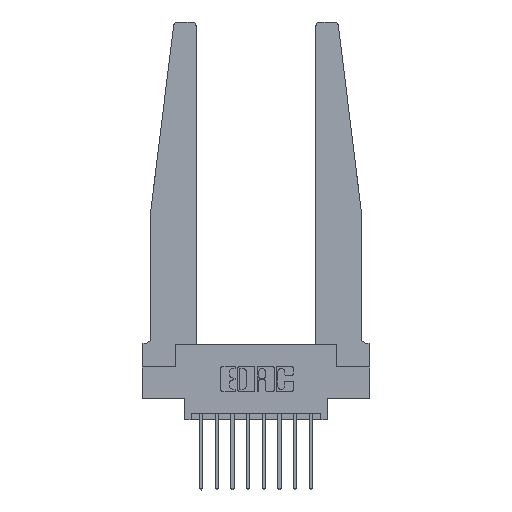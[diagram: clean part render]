
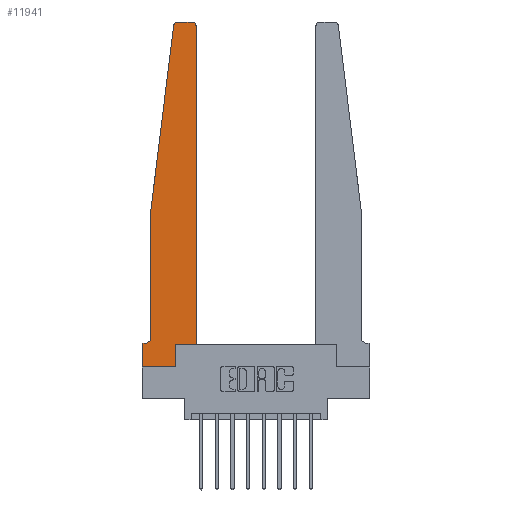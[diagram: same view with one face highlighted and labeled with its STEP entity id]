
A CAD part, top view. The second image highlights one B-rep face of the part: STEP entity #11941.
In plain terms, the highlighted planar face has unit normal (0, 0, 1).
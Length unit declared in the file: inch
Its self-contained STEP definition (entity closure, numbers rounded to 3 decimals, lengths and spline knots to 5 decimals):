
#55 = ORIENTED_EDGE ( 'NONE', *, *, #4437, .T. ) ;
#72 = VECTOR ( 'NONE', #4431, 39.37008 ) ;
#84 = VECTOR ( 'NONE', #1507, 39.37008 ) ;
#110 = CARTESIAN_POINT ( 'NONE',  ( 0.27653, 2.75, 0.37 ) ) ;
#805 = CARTESIAN_POINT ( 'NONE',  ( 0.065, 1.25, 0.37 ) ) ;
#970 = CARTESIAN_POINT ( 'NONE',  ( 0.065, 1.25, 0.37 ) ) ;
#1262 = EDGE_LOOP ( 'NONE', ( #13787, #9319, #13698, #7405, #13806, #8957, #1422, #9100, #9950, #10166, #55, #6758 ) ) ;
#1422 = ORIENTED_EDGE ( 'NONE', *, *, #10849, .T. ) ;
#1507 = DIRECTION ( 'NONE',  ( 0., 1., 0. ) ) ;
#1625 = VERTEX_POINT ( 'NONE', #13181 ) ;
#1698 = EDGE_CURVE ( 'NONE', #13795, #2586, #1751, .T. ) ;
#1751 = CIRCLE ( 'NONE', #6270, 0.05 ) ;
#2132 = AXIS2_PLACEMENT_3D ( 'NONE', #11994, #5197, #13147 ) ;
#2185 = DIRECTION ( 'NONE',  ( -1., 0., 0. ) ) ;
#2275 = LINE ( 'NONE', #2280, #10970 ) ;
#2280 = CARTESIAN_POINT ( 'NONE',  ( 0., 0., 0.37 ) ) ;
#2449 = CARTESIAN_POINT ( 'NONE',  ( 0.2605, 0.18, 0.37 ) ) ;
#2534 = VECTOR ( 'NONE', #2185, 39.37008 ) ;
#2586 = VERTEX_POINT ( 'NONE', #4735 ) ;
#2607 = DIRECTION ( 'NONE',  ( 0., 0., 1. ) ) ;
#2850 = VECTOR ( 'NONE', #12001, 39.37008 ) ;
#2880 = LINE ( 'NONE', #13566, #2534 ) ;
#3452 = CARTESIAN_POINT ( 'NONE',  ( 0., 0., 0.37 ) ) ;
#3646 = CIRCLE ( 'NONE', #10061, 0.03 ) ;
#3880 = CARTESIAN_POINT ( 'NONE',  ( 0., 0., 0.37 ) ) ;
#4180 = EDGE_CURVE ( 'NONE', #2586, #12520, #9156, .T. ) ;
#4248 = DIRECTION ( 'NONE',  ( -0.122, -0.992, 0. ) ) ;
#4431 = DIRECTION ( 'NONE',  ( -1., 0., 0. ) ) ;
#4437 = EDGE_CURVE ( 'NONE', #9619, #8622, #12184, .T. ) ;
#4735 = CARTESIAN_POINT ( 'NONE',  ( 0.015, 0.1875, 0.37 ) ) ;
#4822 = LINE ( 'NONE', #13734, #10512 ) ;
#5020 = DIRECTION ( 'NONE',  ( 0., -1., 0. ) ) ;
#5117 = LINE ( 'NONE', #3880, #11156 ) ;
#5148 = LINE ( 'NONE', #805, #10827 ) ;
#5197 = DIRECTION ( 'NONE',  ( 0., 0., 1. ) ) ;
#5408 = VERTEX_POINT ( 'NONE', #970 ) ;
#5577 = VERTEX_POINT ( 'NONE', #110 ) ;
#5584 = EDGE_CURVE ( 'NONE', #5577, #13607, #3646, .T. ) ;
#5821 = DIRECTION ( 'NONE',  ( 1., 0., 0. ) ) ;
#5870 = LINE ( 'NONE', #10859, #2850 ) ;
#5886 = DIRECTION ( 'NONE',  ( 0., 0., 1. ) ) ;
#6270 = AXIS2_PLACEMENT_3D ( 'NONE', #13327, #6499, #14466 ) ;
#6499 = DIRECTION ( 'NONE',  ( 0., 0., -1. ) ) ;
#6758 = ORIENTED_EDGE ( 'NONE', *, *, #14075, .T. ) ;
#6815 = CARTESIAN_POINT ( 'NONE',  ( 0.2605, 0.18, 0.37 ) ) ;
#6899 = VECTOR ( 'NONE', #8167, 39.37008 ) ;
#7108 = CARTESIAN_POINT ( 'NONE',  ( 0., 0.1875, 0.37 ) ) ;
#7230 = VERTEX_POINT ( 'NONE', #6815 ) ;
#7304 = CIRCLE ( 'NONE', #2132, 0.03 ) ;
#7405 = ORIENTED_EDGE ( 'NONE', *, *, #8548, .T. ) ;
#7636 = EDGE_CURVE ( 'NONE', #7230, #9619, #4822, .T. ) ;
#8167 = DIRECTION ( 'NONE',  ( 0., 1., 0. ) ) ;
#8548 = EDGE_CURVE ( 'NONE', #5408, #13795, #5870, .T. ) ;
#8622 = VERTEX_POINT ( 'NONE', #9868 ) ;
#8688 = AXIS2_PLACEMENT_3D ( 'NONE', #7108, #2607, #10537 ) ;
#8957 = ORIENTED_EDGE ( 'NONE', *, *, #4180, .T. ) ;
#9100 = ORIENTED_EDGE ( 'NONE', *, *, #11100, .T. ) ;
#9156 = LINE ( 'NONE', #12371, #72 ) ;
#9319 = ORIENTED_EDGE ( 'NONE', *, *, #5584, .T. ) ;
#9366 = CARTESIAN_POINT ( 'NONE',  ( 0., 0.1875, 0.37 ) ) ;
#9454 = CARTESIAN_POINT ( 'NONE',  ( 0.425, 0.18, 0.37 ) ) ;
#9619 = VERTEX_POINT ( 'NONE', #14051 ) ;
#9863 = EDGE_CURVE ( 'NONE', #13607, #5408, #5148, .T. ) ;
#9868 = CARTESIAN_POINT ( 'NONE',  ( 0.425, 2.72, 0.37 ) ) ;
#9935 = LINE ( 'NONE', #2449, #6899 ) ;
#9950 = ORIENTED_EDGE ( 'NONE', *, *, #10144, .T. ) ;
#10061 = AXIS2_PLACEMENT_3D ( 'NONE', #12684, #5886, #13843 ) ;
#10066 = FACE_OUTER_BOUND ( 'NONE', #1262, .T. ) ;
#10144 = EDGE_CURVE ( 'NONE', #14463, #7230, #9935, .T. ) ;
#10166 = ORIENTED_EDGE ( 'NONE', *, *, #7636, .T. ) ;
#10221 = DIRECTION ( 'NONE',  ( 1., 0., 0. ) ) ;
#10512 = VECTOR ( 'NONE', #5821, 39.37008 ) ;
#10537 = DIRECTION ( 'NONE',  ( 1., 0., 0. ) ) ;
#10827 = VECTOR ( 'NONE', #4248, 39.37008 ) ;
#10849 = EDGE_CURVE ( 'NONE', #12520, #11759, #5117, .T. ) ;
#10859 = CARTESIAN_POINT ( 'NONE',  ( 0.065, 1.25, 0.37 ) ) ;
#10970 = VECTOR ( 'NONE', #10221, 39.37008 ) ;
#11100 = EDGE_CURVE ( 'NONE', #11759, #14463, #2275, .T. ) ;
#11113 = CARTESIAN_POINT ( 'NONE',  ( 0.24675, 2.72367, 0.37 ) ) ;
#11156 = VECTOR ( 'NONE', #5020, 39.37008 ) ;
#11638 = PLANE ( 'NONE',  #8688 ) ;
#11759 = VERTEX_POINT ( 'NONE', #3452 ) ;
#11941 = ADVANCED_FACE ( 'NONE', ( #10066 ), #11638, .T. ) ;
#11994 = CARTESIAN_POINT ( 'NONE',  ( 0.395, 2.72, 0.37 ) ) ;
#12001 = DIRECTION ( 'NONE',  ( 0., -1., 0. ) ) ;
#12184 = LINE ( 'NONE', #9454, #84 ) ;
#12371 = CARTESIAN_POINT ( 'NONE',  ( 0.065, 0.1875, 0.37 ) ) ;
#12520 = VERTEX_POINT ( 'NONE', #9366 ) ;
#12684 = CARTESIAN_POINT ( 'NONE',  ( 0.27653, 2.72, 0.37 ) ) ;
#12975 = CARTESIAN_POINT ( 'NONE',  ( 0.2605, 0., 0.37 ) ) ;
#13147 = DIRECTION ( 'NONE',  ( 1., 0., 0. ) ) ;
#13181 = CARTESIAN_POINT ( 'NONE',  ( 0.395, 2.75, 0.37 ) ) ;
#13327 = CARTESIAN_POINT ( 'NONE',  ( 0.015, 0.2375, 0.37 ) ) ;
#13566 = CARTESIAN_POINT ( 'NONE',  ( 0.25, 2.75, 0.37 ) ) ;
#13607 = VERTEX_POINT ( 'NONE', #11113 ) ;
#13698 = ORIENTED_EDGE ( 'NONE', *, *, #9863, .T. ) ;
#13707 = CARTESIAN_POINT ( 'NONE',  ( 0.065, 0.2375, 0.37 ) ) ;
#13721 = EDGE_CURVE ( 'NONE', #1625, #5577, #2880, .T. ) ;
#13734 = CARTESIAN_POINT ( 'NONE',  ( 0.425, 0.18, 0.37 ) ) ;
#13787 = ORIENTED_EDGE ( 'NONE', *, *, #13721, .T. ) ;
#13795 = VERTEX_POINT ( 'NONE', #13707 ) ;
#13806 = ORIENTED_EDGE ( 'NONE', *, *, #1698, .T. ) ;
#13843 = DIRECTION ( 'NONE',  ( 1., 0., 0. ) ) ;
#14051 = CARTESIAN_POINT ( 'NONE',  ( 0.425, 0.18, 0.37 ) ) ;
#14075 = EDGE_CURVE ( 'NONE', #8622, #1625, #7304, .T. ) ;
#14463 = VERTEX_POINT ( 'NONE', #12975 ) ;
#14466 = DIRECTION ( 'NONE',  ( -1., 0., 0. ) ) ;
